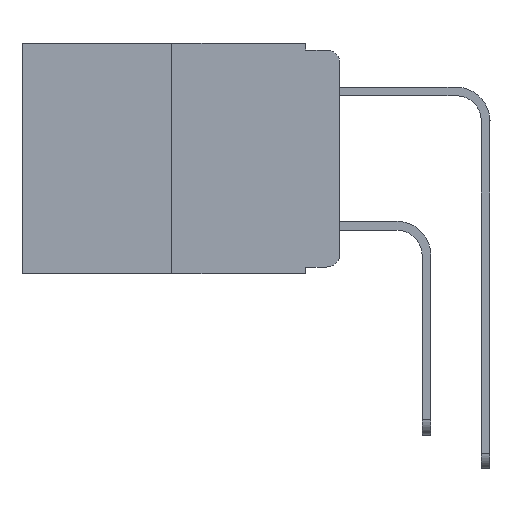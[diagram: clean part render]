
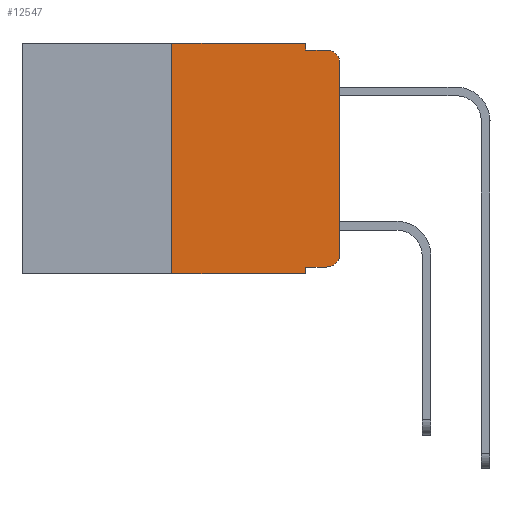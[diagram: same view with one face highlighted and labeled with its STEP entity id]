
A CAD part, left-side view. The second image highlights one B-rep face of the part: STEP entity #12547.
In plain terms, the highlighted planar face has unit normal (-1, 0, 0).
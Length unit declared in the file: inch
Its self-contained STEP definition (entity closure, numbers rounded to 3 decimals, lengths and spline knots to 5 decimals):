
#129 = DIRECTION ( 'NONE',  ( 0., -1., 0. ) ) ;
#163 = EDGE_CURVE ( 'NONE', #22820, #2736, #13346, .T. ) ;
#554 = DIRECTION ( 'NONE',  ( 0., -1., 0. ) ) ;
#623 = VERTEX_POINT ( 'NONE', #12217 ) ;
#2083 = CARTESIAN_POINT ( 'NONE',  ( 0., 0.051, 0. ) ) ;
#2106 = EDGE_CURVE ( 'NONE', #18897, #9300, #8548, .T. ) ;
#2479 = CARTESIAN_POINT ( 'NONE',  ( 0., 0.051, -0.343 ) ) ;
#2736 = VERTEX_POINT ( 'NONE', #10399 ) ;
#3840 = AXIS2_PLACEMENT_3D ( 'NONE', #16419, #5262, #18205 ) ;
#3990 = EDGE_CURVE ( 'NONE', #2736, #18897, #13949, .T. ) ;
#3998 = DIRECTION ( 'NONE',  ( 0., 0., -1. ) ) ;
#4275 = EDGE_CURVE ( 'NONE', #21960, #18596, #20935, .T. ) ;
#4418 = ORIENTED_EDGE ( 'NONE', *, *, #19067, .F. ) ;
#4468 = DIRECTION ( 'NONE',  ( 0., 0., 1. ) ) ;
#4741 = ORIENTED_EDGE ( 'NONE', *, *, #163, .T. ) ;
#5262 = DIRECTION ( 'NONE',  ( -1., 0., 0. ) ) ;
#6534 = ORIENTED_EDGE ( 'NONE', *, *, #10899, .F. ) ;
#6725 = VECTOR ( 'NONE', #554, 39.37008 ) ;
#6841 = ORIENTED_EDGE ( 'NONE', *, *, #22370, .F. ) ;
#6886 = VECTOR ( 'NONE', #7636, 39.37008 ) ;
#7383 = CARTESIAN_POINT ( 'NONE',  ( 0., 0., -0.313 ) ) ;
#7447 = VECTOR ( 'NONE', #9319, 39.37008 ) ;
#7636 = DIRECTION ( 'NONE',  ( 0., -1., 0. ) ) ;
#8270 = CIRCLE ( 'NONE', #3840, 0.02 ) ;
#8441 = VERTEX_POINT ( 'NONE', #21475 ) ;
#8529 = EDGE_CURVE ( 'NONE', #9300, #15097, #8270, .T. ) ;
#8548 = LINE ( 'NONE', #14817, #12921 ) ;
#8752 = LINE ( 'NONE', #18817, #22065 ) ;
#9300 = VERTEX_POINT ( 'NONE', #15034 ) ;
#9319 = DIRECTION ( 'NONE',  ( 0., 0., 1. ) ) ;
#9723 = DIRECTION ( 'NONE',  ( -1., 0., 0. ) ) ;
#9732 = CARTESIAN_POINT ( 'NONE',  ( 0., 0.051, -0.333 ) ) ;
#10266 = VECTOR ( 'NONE', #3998, 39.37008 ) ;
#10399 = CARTESIAN_POINT ( 'NONE',  ( 0., 0.02, -0.333 ) ) ;
#10784 = DIRECTION ( 'NONE',  ( 0., 0., -1. ) ) ;
#10899 = EDGE_CURVE ( 'NONE', #623, #15097, #20882, .T. ) ;
#11535 = FACE_OUTER_BOUND ( 'NONE', #23086, .T. ) ;
#11657 = DIRECTION ( 'NONE',  ( 0., 0., -1. ) ) ;
#11743 = LINE ( 'NONE', #11969, #6725 ) ;
#11769 = VERTEX_POINT ( 'NONE', #2479 ) ;
#11848 = LINE ( 'NONE', #20182, #7447 ) ;
#11969 = CARTESIAN_POINT ( 'NONE',  ( 0., 0.473, -0.343 ) ) ;
#12083 = CARTESIAN_POINT ( 'NONE',  ( 0., 0.051, 0. ) ) ;
#12217 = CARTESIAN_POINT ( 'NONE',  ( 0., 0.051, -0.01 ) ) ;
#12547 = ADVANCED_FACE ( 'NONE', ( #11535 ), #23217, .F. ) ;
#12921 = VECTOR ( 'NONE', #4468, 39.37008 ) ;
#13008 = ORIENTED_EDGE ( 'NONE', *, *, #18068, .T. ) ;
#13346 = LINE ( 'NONE', #9732, #22280 ) ;
#13949 = CIRCLE ( 'NONE', #23080, 0.02 ) ;
#14125 = AXIS2_PLACEMENT_3D ( 'NONE', #19762, #21567, #10784 ) ;
#14138 = CARTESIAN_POINT ( 'NONE',  ( 0., 0.473, 0. ) ) ;
#14817 = CARTESIAN_POINT ( 'NONE',  ( 0., 0., 0. ) ) ;
#15034 = CARTESIAN_POINT ( 'NONE',  ( 0., 0., -0.03 ) ) ;
#15097 = VERTEX_POINT ( 'NONE', #22762 ) ;
#15818 = ORIENTED_EDGE ( 'NONE', *, *, #2106, .T. ) ;
#16054 = CARTESIAN_POINT ( 'NONE',  ( 0., 0.051, -0.333 ) ) ;
#16223 = VECTOR ( 'NONE', #21335, 39.37008 ) ;
#16419 = CARTESIAN_POINT ( 'NONE',  ( 0., 0.02, -0.03 ) ) ;
#16678 = ORIENTED_EDGE ( 'NONE', *, *, #4275, .F. ) ;
#17936 = EDGE_CURVE ( 'NONE', #22820, #11769, #19899, .T. ) ;
#18048 = ORIENTED_EDGE ( 'NONE', *, *, #8529, .T. ) ;
#18068 = EDGE_CURVE ( 'NONE', #8441, #11769, #11743, .T. ) ;
#18205 = DIRECTION ( 'NONE',  ( 0., 0., -1. ) ) ;
#18594 = CARTESIAN_POINT ( 'NONE',  ( 0., 0.051, -0.01 ) ) ;
#18596 = VERTEX_POINT ( 'NONE', #12083 ) ;
#18817 = CARTESIAN_POINT ( 'NONE',  ( 0., 0.051, 0. ) ) ;
#18897 = VERTEX_POINT ( 'NONE', #7383 ) ;
#19067 = EDGE_CURVE ( 'NONE', #18596, #623, #8752, .T. ) ;
#19762 = CARTESIAN_POINT ( 'NONE',  ( 0., 0.473, 0. ) ) ;
#19899 = LINE ( 'NONE', #2083, #10266 ) ;
#20182 = CARTESIAN_POINT ( 'NONE',  ( 0., 0.25, 0. ) ) ;
#20557 = CARTESIAN_POINT ( 'NONE',  ( 0., 0.02, -0.313 ) ) ;
#20882 = LINE ( 'NONE', #18594, #6886 ) ;
#20935 = LINE ( 'NONE', #14138, #16223 ) ;
#21335 = DIRECTION ( 'NONE',  ( 0., -1., 0. ) ) ;
#21475 = CARTESIAN_POINT ( 'NONE',  ( 0., 0.25, -0.343 ) ) ;
#21567 = DIRECTION ( 'NONE',  ( 1., 0., 0. ) ) ;
#21948 = ORIENTED_EDGE ( 'NONE', *, *, #17936, .F. ) ;
#21960 = VERTEX_POINT ( 'NONE', #22354 ) ;
#22065 = VECTOR ( 'NONE', #11657, 39.37008 ) ;
#22280 = VECTOR ( 'NONE', #129, 39.37008 ) ;
#22329 = DIRECTION ( 'NONE',  ( 0., 0., -1. ) ) ;
#22354 = CARTESIAN_POINT ( 'NONE',  ( 0., 0.25, 0. ) ) ;
#22370 = EDGE_CURVE ( 'NONE', #8441, #21960, #11848, .T. ) ;
#22762 = CARTESIAN_POINT ( 'NONE',  ( 0., 0.02, -0.01 ) ) ;
#22820 = VERTEX_POINT ( 'NONE', #16054 ) ;
#23080 = AXIS2_PLACEMENT_3D ( 'NONE', #20557, #9723, #22329 ) ;
#23086 = EDGE_LOOP ( 'NONE', ( #15818, #18048, #6534, #4418, #16678, #6841, #13008, #21948, #4741, #23305 ) ) ;
#23217 = PLANE ( 'NONE',  #14125 ) ;
#23305 = ORIENTED_EDGE ( 'NONE', *, *, #3990, .T. ) ;
